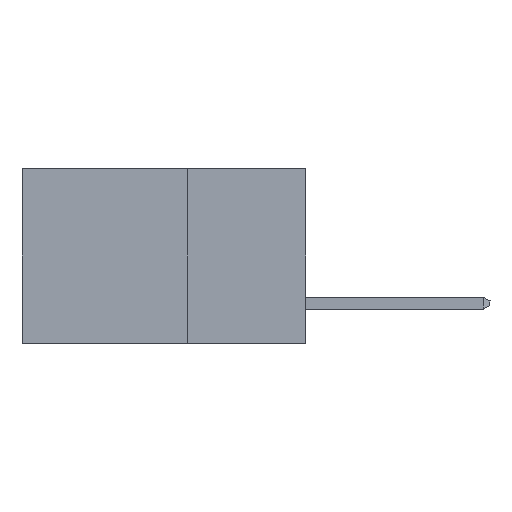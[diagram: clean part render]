
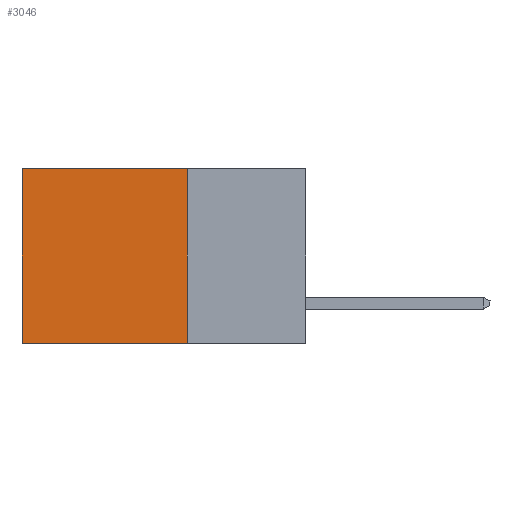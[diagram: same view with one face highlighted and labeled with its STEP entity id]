
A CAD part, left-side view. The second image highlights one B-rep face of the part: STEP entity #3046.
In plain terms, the highlighted planar face has unit normal (-1, 0, 0).
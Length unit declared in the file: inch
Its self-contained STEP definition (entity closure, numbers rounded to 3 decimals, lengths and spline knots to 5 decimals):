
#832 = CARTESIAN_POINT ( 'NONE',  ( 0.298, 0.6, 0. ) ) ;
#1189 = VECTOR ( 'NONE', #11147, 39.37008 ) ;
#1516 = ORIENTED_EDGE ( 'NONE', *, *, #7535, .T. ) ;
#2106 = DIRECTION ( 'NONE',  ( 0., 0., -1. ) ) ;
#3026 = CARTESIAN_POINT ( 'NONE',  ( 0.298, 0.25, 0. ) ) ;
#3046 = ADVANCED_FACE ( 'NONE', ( #12446 ), #4388, .F. ) ;
#3152 = VERTEX_POINT ( 'NONE', #3347 ) ;
#3347 = CARTESIAN_POINT ( 'NONE',  ( 0.298, 0.25, -0.37 ) ) ;
#4388 = PLANE ( 'NONE',  #5776 ) ;
#4571 = ORIENTED_EDGE ( 'NONE', *, *, #16723, .F. ) ;
#5188 = CARTESIAN_POINT ( 'NONE',  ( 0.298, 0.25, -0.37 ) ) ;
#5771 = VECTOR ( 'NONE', #16991, 39.37008 ) ;
#5776 = AXIS2_PLACEMENT_3D ( 'NONE', #3026, #5870, #11207 ) ;
#5870 = DIRECTION ( 'NONE',  ( 1., 0., 0. ) ) ;
#6020 = LINE ( 'NONE', #18535, #1189 ) ;
#6351 = EDGE_LOOP ( 'NONE', ( #1516, #4571, #9676, #13318 ) ) ;
#6646 = LINE ( 'NONE', #16743, #14216 ) ;
#7180 = CARTESIAN_POINT ( 'NONE',  ( 0.298, 0.6, -0.37 ) ) ;
#7204 = CARTESIAN_POINT ( 'NONE',  ( 0.298, 0.6, 0. ) ) ;
#7471 = VECTOR ( 'NONE', #8251, 39.37008 ) ;
#7535 = EDGE_CURVE ( 'NONE', #14686, #8164, #17693, .T. ) ;
#8164 = VERTEX_POINT ( 'NONE', #7180 ) ;
#8251 = DIRECTION ( 'NONE',  ( 0., 1., 0. ) ) ;
#9676 = ORIENTED_EDGE ( 'NONE', *, *, #11192, .F. ) ;
#11147 = DIRECTION ( 'NONE',  ( 0., 1., 0. ) ) ;
#11192 = EDGE_CURVE ( 'NONE', #16124, #3152, #6646, .T. ) ;
#11207 = DIRECTION ( 'NONE',  ( 0., 0., -1. ) ) ;
#12446 = FACE_OUTER_BOUND ( 'NONE', #6351, .T. ) ;
#13318 = ORIENTED_EDGE ( 'NONE', *, *, #18764, .T. ) ;
#13795 = CARTESIAN_POINT ( 'NONE',  ( 0.298, 0.25, 0. ) ) ;
#14216 = VECTOR ( 'NONE', #2106, 39.37008 ) ;
#14686 = VERTEX_POINT ( 'NONE', #7204 ) ;
#16124 = VERTEX_POINT ( 'NONE', #13795 ) ;
#16723 = EDGE_CURVE ( 'NONE', #3152, #8164, #17985, .T. ) ;
#16743 = CARTESIAN_POINT ( 'NONE',  ( 0.298, 0.25, 0. ) ) ;
#16991 = DIRECTION ( 'NONE',  ( 0., 0., -1. ) ) ;
#17693 = LINE ( 'NONE', #832, #5771 ) ;
#17985 = LINE ( 'NONE', #5188, #7471 ) ;
#18535 = CARTESIAN_POINT ( 'NONE',  ( 0.298, 0.25, 0. ) ) ;
#18764 = EDGE_CURVE ( 'NONE', #16124, #14686, #6020, .T. ) ;
